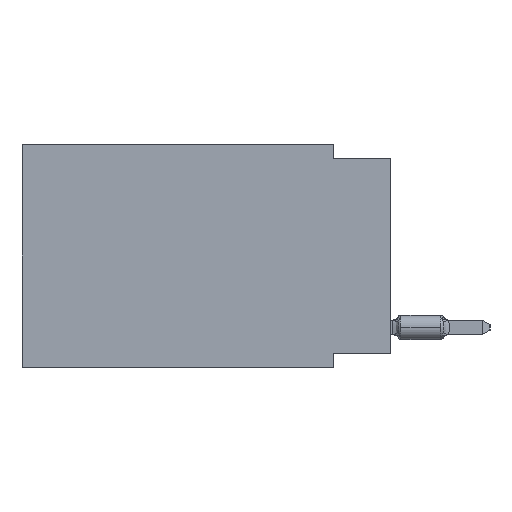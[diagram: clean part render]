
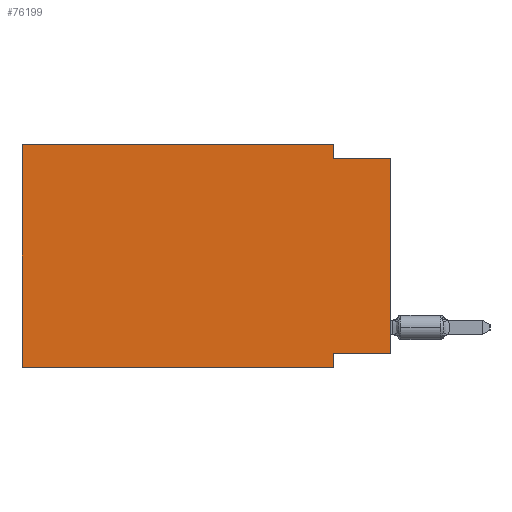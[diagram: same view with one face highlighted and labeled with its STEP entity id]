
A CAD part, left-side view. The second image highlights one B-rep face of the part: STEP entity #76199.
In plain terms, the highlighted planar face has unit normal (-1, 0, 0).
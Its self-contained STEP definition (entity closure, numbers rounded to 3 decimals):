
#740 = EDGE_CURVE ( 'NONE', #13439, #30097, #76745, .T. ) ;
#3348 = VERTEX_POINT ( 'NONE', #57824 ) ;
#3389 = EDGE_CURVE ( 'NONE', #71291, #61477, #4002, .T. ) ;
#3610 = DIRECTION ( 'NONE',  ( 0., 0., 1. ) ) ;
#3926 = ORIENTED_EDGE ( 'NONE', *, *, #7764, .F. ) ;
#3995 = DIRECTION ( 'NONE',  ( 1., 0., 0. ) ) ;
#4002 = LINE ( 'NONE', #27788, #47252 ) ;
#4764 = DIRECTION ( 'NONE',  ( 0., 0., -1. ) ) ;
#5743 = EDGE_LOOP ( 'NONE', ( #19264, #3926, #61381, #26191, #16285, #51252, #24882, #15160 ) ) ;
#7764 = EDGE_CURVE ( 'NONE', #38120, #44965, #24687, .T. ) ;
#7917 = EDGE_CURVE ( 'NONE', #13439, #44965, #69145, .T. ) ;
#9794 = DIRECTION ( 'NONE',  ( 0., 0., -1. ) ) ;
#11334 = DIRECTION ( 'NONE',  ( 0., 0., 1. ) ) ;
#13439 = VERTEX_POINT ( 'NONE', #74450 ) ;
#14168 = DIRECTION ( 'NONE',  ( 0., 0., -1. ) ) ;
#15160 = ORIENTED_EDGE ( 'NONE', *, *, #740, .F. ) ;
#15445 = EDGE_CURVE ( 'NONE', #3348, #36153, #64639, .T. ) ;
#16077 = CARTESIAN_POINT ( 'NONE',  ( 0., 16.383, 0. ) ) ;
#16145 = EDGE_CURVE ( 'NONE', #61477, #38120, #68400, .T. ) ;
#16285 = ORIENTED_EDGE ( 'NONE', *, *, #72546, .F. ) ;
#18127 = CARTESIAN_POINT ( 'NONE',  ( 0., 2.54, -9.271 ) ) ;
#18151 = VECTOR ( 'NONE', #52926, 1000. ) ;
#19264 = ORIENTED_EDGE ( 'NONE', *, *, #7917, .T. ) ;
#19982 = CARTESIAN_POINT ( 'NONE',  ( 0., 0., -0.635 ) ) ;
#20534 = VECTOR ( 'NONE', #3610, 1000. ) ;
#21096 = CARTESIAN_POINT ( 'NONE',  ( 0., 2.54, -9.906 ) ) ;
#24025 = DIRECTION ( 'NONE',  ( 0., 1., 0. ) ) ;
#24687 = LINE ( 'NONE', #19982, #55204 ) ;
#24882 = ORIENTED_EDGE ( 'NONE', *, *, #75540, .F. ) ;
#26191 = ORIENTED_EDGE ( 'NONE', *, *, #3389, .F. ) ;
#27788 = CARTESIAN_POINT ( 'NONE',  ( 0., 16.383, 0. ) ) ;
#30097 = VERTEX_POINT ( 'NONE', #18127 ) ;
#32866 = CARTESIAN_POINT ( 'NONE',  ( 0., 0., 0. ) ) ;
#35880 = CARTESIAN_POINT ( 'NONE',  ( 0., 16.383, 0. ) ) ;
#36153 = VERTEX_POINT ( 'NONE', #75460 ) ;
#37578 = CARTESIAN_POINT ( 'NONE',  ( 0., 2.54, 0. ) ) ;
#38120 = VERTEX_POINT ( 'NONE', #49400 ) ;
#39071 = CARTESIAN_POINT ( 'NONE',  ( 0., 16.383, 0. ) ) ;
#40264 = VECTOR ( 'NONE', #11334, 1000. ) ;
#40697 = CARTESIAN_POINT ( 'NONE',  ( 0., 0., -0.635 ) ) ;
#40840 = CARTESIAN_POINT ( 'NONE',  ( 0., 0., -9.271 ) ) ;
#44965 = VERTEX_POINT ( 'NONE', #40697 ) ;
#47252 = VECTOR ( 'NONE', #75399, 1000. ) ;
#49400 = CARTESIAN_POINT ( 'NONE',  ( 0., 2.54, -0.635 ) ) ;
#50746 = LINE ( 'NONE', #21096, #61795 ) ;
#51006 = CARTESIAN_POINT ( 'NONE',  ( 0., 2.54, 0. ) ) ;
#51252 = ORIENTED_EDGE ( 'NONE', *, *, #15445, .T. ) ;
#51584 = FACE_OUTER_BOUND ( 'NONE', #5743, .T. ) ;
#52058 = VECTOR ( 'NONE', #24025, 1000. ) ;
#52926 = DIRECTION ( 'NONE',  ( 0., -1., 0. ) ) ;
#54344 = AXIS2_PLACEMENT_3D ( 'NONE', #16077, #3995, #4764 ) ;
#55204 = VECTOR ( 'NONE', #66442, 1000. ) ;
#57824 = CARTESIAN_POINT ( 'NONE',  ( 0., 16.383, -9.906 ) ) ;
#61381 = ORIENTED_EDGE ( 'NONE', *, *, #16145, .F. ) ;
#61477 = VERTEX_POINT ( 'NONE', #51006 ) ;
#61795 = VECTOR ( 'NONE', #9794, 1000. ) ;
#64255 = CARTESIAN_POINT ( 'NONE',  ( 0., 16.383, -9.906 ) ) ;
#64639 = LINE ( 'NONE', #64255, #18151 ) ;
#65194 = PLANE ( 'NONE',  #54344 ) ;
#65669 = VECTOR ( 'NONE', #14168, 1000. ) ;
#66316 = LINE ( 'NONE', #35880, #40264 ) ;
#66442 = DIRECTION ( 'NONE',  ( 0., -1., 0. ) ) ;
#68400 = LINE ( 'NONE', #37578, #65669 ) ;
#69145 = LINE ( 'NONE', #32866, #20534 ) ;
#71291 = VERTEX_POINT ( 'NONE', #39071 ) ;
#72546 = EDGE_CURVE ( 'NONE', #3348, #71291, #66316, .T. ) ;
#74450 = CARTESIAN_POINT ( 'NONE',  ( 0., 0., -9.271 ) ) ;
#75399 = DIRECTION ( 'NONE',  ( 0., -1., 0. ) ) ;
#75460 = CARTESIAN_POINT ( 'NONE',  ( 0., 2.54, -9.906 ) ) ;
#75540 = EDGE_CURVE ( 'NONE', #30097, #36153, #50746, .T. ) ;
#76199 = ADVANCED_FACE ( 'NONE', ( #51584 ), #65194, .F. ) ;
#76745 = LINE ( 'NONE', #40840, #52058 ) ;
